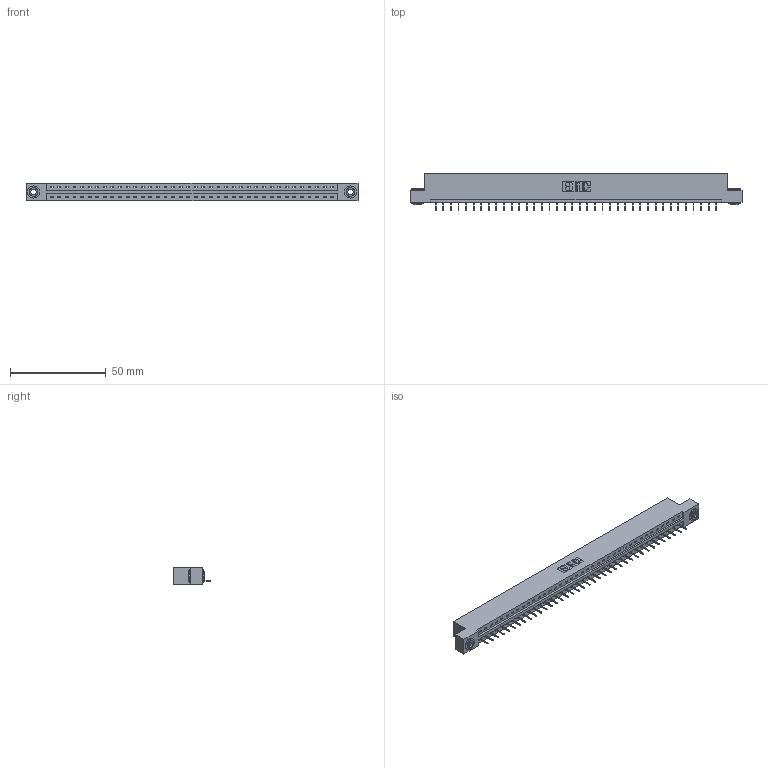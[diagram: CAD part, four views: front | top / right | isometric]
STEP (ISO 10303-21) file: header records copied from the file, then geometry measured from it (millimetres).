
FILE_DESCRIPTION (( 'STEP AP203' ), '1' );
FILE_NAME ('387-038-524-103.STEP', '2019-10-04T15:48:09', ( '' ), ( '' ), 'SwSTEP 2.0', 'SolidWorks 2016', '' );
FILE_SCHEMA (( 'CONFIG_CONTROL_DESIGN' ));
Length unit declared in the file: inch
Products named in the file (4): 345-292-001_345-293-124; 345-250-002_345-250-002-102; 337 Part_Flush Mounting Lugs - 0.156 Dia-TH; 387-038-524-103
Assembly tree (41 placements, depth 2):
  387-038-524-103
    337 Part_Flush Mounting Lugs - 0.156 Dia-TH
    345-292-001_345-293-124  x38
    345-250-002_345-250-002-102  x2
Bounding box: 173.58 x 19.69 x 9.4 mm (x, y, z)
Volume: 17860.3 mm3; surface area: 18138.6 mm2
Topology: 41 solids, 41 shells, 2660 faces, 7683 edges, 4966 vertices
Faces by surface type: plane 2056, cylinder 596, cone 8
Entity records: 29488 total; most frequent: CARTESIAN_POINT 5111, ORIENTED_EDGE 5078, DIRECTION 4345, EDGE_CURVE 2539, LINE 2391, VECTOR 2391, VERTEX_POINT 1686, AXIS2_PLACEMENT_3D 977
